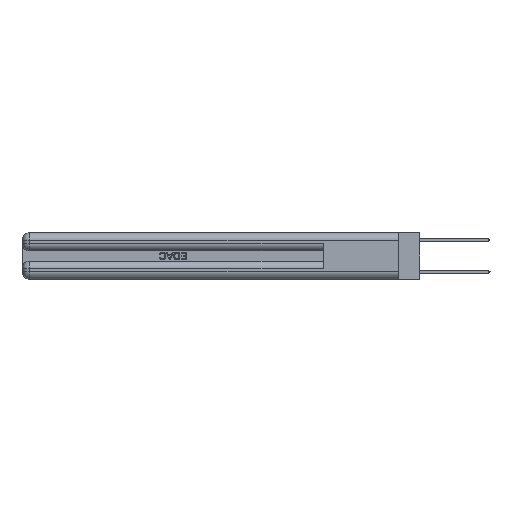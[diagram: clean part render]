
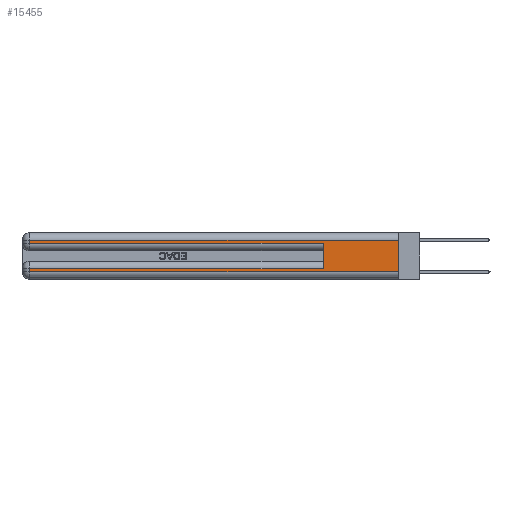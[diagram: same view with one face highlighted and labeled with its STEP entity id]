
A CAD part, left-side view. The second image highlights one B-rep face of the part: STEP entity #15455.
In plain terms, the highlighted planar face has unit normal (-1, 0, 0).
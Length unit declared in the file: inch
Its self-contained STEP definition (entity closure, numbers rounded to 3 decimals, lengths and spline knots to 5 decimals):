
#599 = EDGE_CURVE ( 'NONE', #31099, #20705, #11654, .T. ) ;
#652 = CARTESIAN_POINT ( 'NONE',  ( 0., 0., 0.06 ) ) ;
#843 = EDGE_CURVE ( 'NONE', #31099, #11664, #5703, .T. ) ;
#1165 = CARTESIAN_POINT ( 'NONE',  ( 0., 2.94, 0.285 ) ) ;
#1433 = EDGE_CURVE ( 'NONE', #32309, #13758, #17940, .T. ) ;
#2681 = LINE ( 'NONE', #25756, #16066 ) ;
#2705 = CARTESIAN_POINT ( 'NONE',  ( 0., 2.94, 0.085 ) ) ;
#3681 = CARTESIAN_POINT ( 'NONE',  ( 0., 0., 0.085 ) ) ;
#4568 = ORIENTED_EDGE ( 'NONE', *, *, #843, .F. ) ;
#4596 = EDGE_CURVE ( 'NONE', #27958, #11664, #14802, .T. ) ;
#4648 = ORIENTED_EDGE ( 'NONE', *, *, #13203, .F. ) ;
#4847 = VERTEX_POINT ( 'NONE', #34208 ) ;
#5002 = DIRECTION ( 'NONE',  ( 0., 0., -1. ) ) ;
#5703 = LINE ( 'NONE', #34807, #10887 ) ;
#6543 = FACE_OUTER_BOUND ( 'NONE', #25970, .T. ) ;
#8016 = VECTOR ( 'NONE', #18344, 39.37008 ) ;
#9269 = CARTESIAN_POINT ( 'NONE',  ( 0., 0.6, 0.145 ) ) ;
#9820 = CARTESIAN_POINT ( 'NONE',  ( 0., 2.94, 0.06 ) ) ;
#10887 = VECTOR ( 'NONE', #5002, 39.37008 ) ;
#11553 = VECTOR ( 'NONE', #35412, 39.37008 ) ;
#11654 = LINE ( 'NONE', #14853, #22974 ) ;
#11664 = VERTEX_POINT ( 'NONE', #652 ) ;
#11771 = EDGE_CURVE ( 'NONE', #4847, #36685, #18038, .T. ) ;
#13203 = EDGE_CURVE ( 'NONE', #4847, #13758, #35540, .T. ) ;
#13248 = ORIENTED_EDGE ( 'NONE', *, *, #599, .T. ) ;
#13758 = VERTEX_POINT ( 'NONE', #22031 ) ;
#14479 = EDGE_CURVE ( 'NONE', #36685, #27958, #2681, .T. ) ;
#14802 = LINE ( 'NONE', #23923, #11553 ) ;
#14853 = CARTESIAN_POINT ( 'NONE',  ( 0., 0., 0.31 ) ) ;
#15036 = PLANE ( 'NONE',  #20276 ) ;
#15189 = DIRECTION ( 'NONE',  ( 0., 1., 0. ) ) ;
#15455 = ADVANCED_FACE ( 'NONE', ( #6543 ), #15036, .F. ) ;
#15475 = DIRECTION ( 'NONE',  ( 0., -1., 0. ) ) ;
#16066 = VECTOR ( 'NONE', #37268, 39.37008 ) ;
#17687 = DIRECTION ( 'NONE',  ( 1., 0., 0. ) ) ;
#17705 = DIRECTION ( 'NONE',  ( 0., 0., -1. ) ) ;
#17940 = LINE ( 'NONE', #32677, #29670 ) ;
#18038 = LINE ( 'NONE', #3681, #26561 ) ;
#18334 = ORIENTED_EDGE ( 'NONE', *, *, #14479, .T. ) ;
#18344 = DIRECTION ( 'NONE',  ( 0., 0., 1. ) ) ;
#20276 = AXIS2_PLACEMENT_3D ( 'NONE', #34707, #17687, #32244 ) ;
#20705 = VERTEX_POINT ( 'NONE', #35828 ) ;
#20726 = DIRECTION ( 'NONE',  ( 0., 1., 0. ) ) ;
#22031 = CARTESIAN_POINT ( 'NONE',  ( 0., 0.6, 0.285 ) ) ;
#22494 = ORIENTED_EDGE ( 'NONE', *, *, #4596, .T. ) ;
#22810 = ORIENTED_EDGE ( 'NONE', *, *, #11771, .T. ) ;
#22974 = VECTOR ( 'NONE', #20726, 39.37008 ) ;
#23923 = CARTESIAN_POINT ( 'NONE',  ( 0., 0., 0.06 ) ) ;
#25756 = CARTESIAN_POINT ( 'NONE',  ( 0., 2.94, 0.37 ) ) ;
#25970 = EDGE_LOOP ( 'NONE', ( #4568, #13248, #32653, #26526, #4648, #22810, #18334, #22494 ) ) ;
#26235 = LINE ( 'NONE', #35798, #27433 ) ;
#26526 = ORIENTED_EDGE ( 'NONE', *, *, #1433, .T. ) ;
#26561 = VECTOR ( 'NONE', #15189, 39.37008 ) ;
#27433 = VECTOR ( 'NONE', #17705, 39.37008 ) ;
#27958 = VERTEX_POINT ( 'NONE', #9820 ) ;
#29506 = CARTESIAN_POINT ( 'NONE',  ( 0., 0., 0.31 ) ) ;
#29670 = VECTOR ( 'NONE', #15475, 39.37008 ) ;
#31099 = VERTEX_POINT ( 'NONE', #29506 ) ;
#32244 = DIRECTION ( 'NONE',  ( 0., 0., -1. ) ) ;
#32309 = VERTEX_POINT ( 'NONE', #1165 ) ;
#32653 = ORIENTED_EDGE ( 'NONE', *, *, #36430, .T. ) ;
#32677 = CARTESIAN_POINT ( 'NONE',  ( 0., 0., 0.285 ) ) ;
#34208 = CARTESIAN_POINT ( 'NONE',  ( 0., 0.6, 0.085 ) ) ;
#34707 = CARTESIAN_POINT ( 'NONE',  ( 0., 0., 0.37 ) ) ;
#34807 = CARTESIAN_POINT ( 'NONE',  ( 0., 0., 0.37 ) ) ;
#35412 = DIRECTION ( 'NONE',  ( 0., -1., 0. ) ) ;
#35540 = LINE ( 'NONE', #9269, #8016 ) ;
#35798 = CARTESIAN_POINT ( 'NONE',  ( 0., 2.94, 0.37 ) ) ;
#35828 = CARTESIAN_POINT ( 'NONE',  ( 0., 2.94, 0.31 ) ) ;
#36430 = EDGE_CURVE ( 'NONE', #20705, #32309, #26235, .T. ) ;
#36685 = VERTEX_POINT ( 'NONE', #2705 ) ;
#37268 = DIRECTION ( 'NONE',  ( 0., 0., -1. ) ) ;
